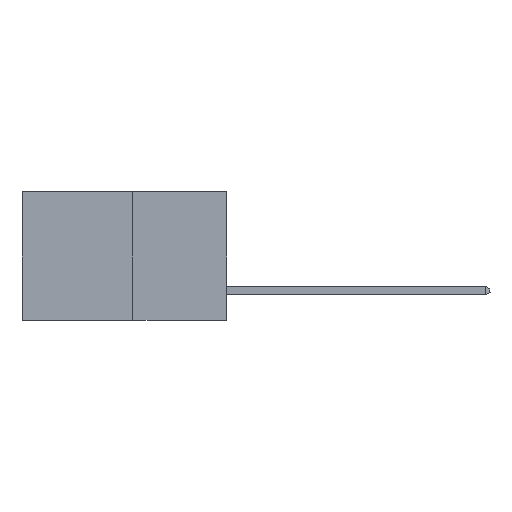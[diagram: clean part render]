
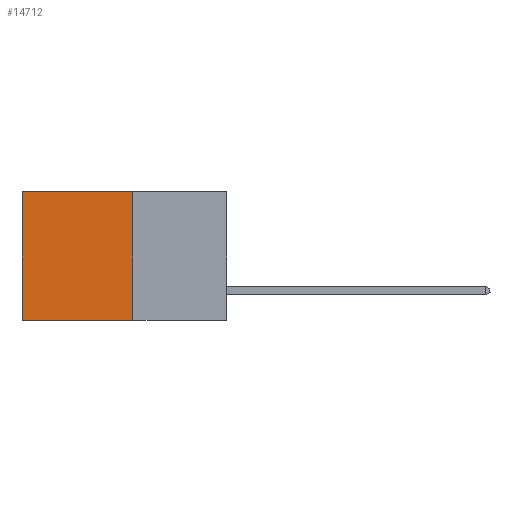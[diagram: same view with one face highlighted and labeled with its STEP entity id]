
A CAD part, left-side view. The second image highlights one B-rep face of the part: STEP entity #14712.
In plain terms, the highlighted planar face has unit normal (-1, 0, 0).
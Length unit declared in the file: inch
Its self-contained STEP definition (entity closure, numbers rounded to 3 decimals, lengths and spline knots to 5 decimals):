
#198 = VERTEX_POINT ( 'NONE', #25419 ) ;
#939 = VECTOR ( 'NONE', #16588, 39.37008 ) ;
#1646 = DIRECTION ( 'NONE',  ( 0., 0., -1. ) ) ;
#1783 = DIRECTION ( 'NONE',  ( 0., 0., -1. ) ) ;
#2978 = VECTOR ( 'NONE', #1783, 39.37008 ) ;
#3843 = LINE ( 'NONE', #26631, #14596 ) ;
#4027 = EDGE_LOOP ( 'NONE', ( #5510, #14963, #26709, #20129 ) ) ;
#4907 = EDGE_CURVE ( 'NONE', #198, #25453, #11400, .T. ) ;
#5148 = VERTEX_POINT ( 'NONE', #21439 ) ;
#5510 = ORIENTED_EDGE ( 'NONE', *, *, #25578, .T. ) ;
#5534 = VECTOR ( 'NONE', #12939, 39.37008 ) ;
#6168 = FACE_OUTER_BOUND ( 'NONE', #4027, .T. ) ;
#6752 = CARTESIAN_POINT ( 'NONE',  ( 0.277, 0.27, -0.37 ) ) ;
#9990 = CARTESIAN_POINT ( 'NONE',  ( 0.277, 0.59, 0. ) ) ;
#11192 = DIRECTION ( 'NONE',  ( 0., 0., -1. ) ) ;
#11400 = LINE ( 'NONE', #14774, #5534 ) ;
#12070 = EDGE_CURVE ( 'NONE', #5148, #24648, #16654, .T. ) ;
#12939 = DIRECTION ( 'NONE',  ( 0., 1., 0. ) ) ;
#14596 = VECTOR ( 'NONE', #1646, 39.37008 ) ;
#14658 = CARTESIAN_POINT ( 'NONE',  ( 0.277, 0.27, -0.37 ) ) ;
#14712 = ADVANCED_FACE ( 'NONE', ( #6168 ), #21420, .F. ) ;
#14774 = CARTESIAN_POINT ( 'NONE',  ( 0.277, 0.27, 0. ) ) ;
#14963 = ORIENTED_EDGE ( 'NONE', *, *, #12070, .F. ) ;
#16588 = DIRECTION ( 'NONE',  ( 0., 1., 0. ) ) ;
#16654 = LINE ( 'NONE', #26698, #939 ) ;
#20129 = ORIENTED_EDGE ( 'NONE', *, *, #4907, .T. ) ;
#20465 = EDGE_CURVE ( 'NONE', #198, #5148, #25221, .T. ) ;
#21420 = PLANE ( 'NONE',  #24144 ) ;
#21439 = CARTESIAN_POINT ( 'NONE',  ( 0.277, 0.27, -0.37 ) ) ;
#23311 = CARTESIAN_POINT ( 'NONE',  ( 0.277, 0.59, -0.37 ) ) ;
#23417 = DIRECTION ( 'NONE',  ( 1., 0., 0. ) ) ;
#24144 = AXIS2_PLACEMENT_3D ( 'NONE', #6752, #23417, #11192 ) ;
#24648 = VERTEX_POINT ( 'NONE', #23311 ) ;
#25221 = LINE ( 'NONE', #14658, #2978 ) ;
#25419 = CARTESIAN_POINT ( 'NONE',  ( 0.277, 0.27, 0. ) ) ;
#25453 = VERTEX_POINT ( 'NONE', #9990 ) ;
#25578 = EDGE_CURVE ( 'NONE', #25453, #24648, #3843, .T. ) ;
#26631 = CARTESIAN_POINT ( 'NONE',  ( 0.277, 0.59, -0.37 ) ) ;
#26698 = CARTESIAN_POINT ( 'NONE',  ( 0.277, 0.27, -0.37 ) ) ;
#26709 = ORIENTED_EDGE ( 'NONE', *, *, #20465, .F. ) ;
